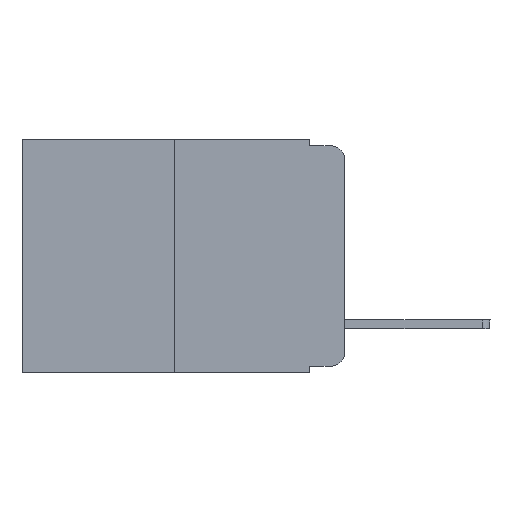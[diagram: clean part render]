
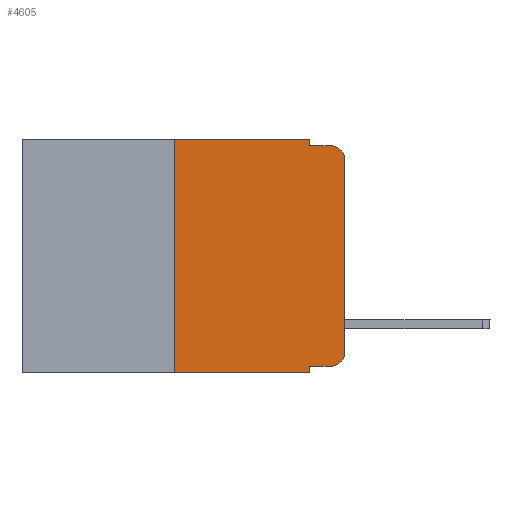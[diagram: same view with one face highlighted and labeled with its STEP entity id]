
A CAD part, left-side view. The second image highlights one B-rep face of the part: STEP entity #4605.
In plain terms, the highlighted planar face has unit normal (-1, 0, 0).
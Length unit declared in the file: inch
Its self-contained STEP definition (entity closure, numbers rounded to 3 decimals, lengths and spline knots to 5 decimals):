
#246 = CIRCLE ( 'NONE', #8995, 0.02 ) ;
#788 = LINE ( 'NONE', #16723, #5142 ) ;
#1160 = CARTESIAN_POINT ( 'NONE',  ( 0., 0.02, -0.01 ) ) ;
#1347 = AXIS2_PLACEMENT_3D ( 'NONE', #11598, #9607, #18611 ) ;
#1408 = FACE_OUTER_BOUND ( 'NONE', #2251, .T. ) ;
#1621 = CARTESIAN_POINT ( 'NONE',  ( 0., 0.25, 0. ) ) ;
#1906 = VECTOR ( 'NONE', #4057, 39.37008 ) ;
#2251 = EDGE_LOOP ( 'NONE', ( #18524, #17222, #21481, #17770, #9551, #10128, #10419, #15243, #20229, #13211 ) ) ;
#2508 = VECTOR ( 'NONE', #10291, 39.37008 ) ;
#2609 = DIRECTION ( 'NONE',  ( 0., 0., -1. ) ) ;
#3590 = VECTOR ( 'NONE', #8158, 39.37008 ) ;
#3754 = DIRECTION ( 'NONE',  ( -1., 0., 0. ) ) ;
#3791 = VERTEX_POINT ( 'NONE', #1160 ) ;
#4057 = DIRECTION ( 'NONE',  ( 0., -1., 0. ) ) ;
#4259 = VERTEX_POINT ( 'NONE', #8747 ) ;
#4409 = VECTOR ( 'NONE', #15600, 39.37008 ) ;
#4416 = LINE ( 'NONE', #5981, #1906 ) ;
#4605 = ADVANCED_FACE ( 'NONE', ( #1408 ), #8684, .F. ) ;
#4695 = LINE ( 'NONE', #9838, #3590 ) ;
#5142 = VECTOR ( 'NONE', #13490, 39.37008 ) ;
#5981 = CARTESIAN_POINT ( 'NONE',  ( 0., 0.051, -0.01 ) ) ;
#6121 = DIRECTION ( 'NONE',  ( 0., -1., 0. ) ) ;
#6798 = CARTESIAN_POINT ( 'NONE',  ( 0., 0.051, -0.01 ) ) ;
#7485 = VERTEX_POINT ( 'NONE', #21274 ) ;
#7593 = EDGE_CURVE ( 'NONE', #18343, #19414, #18879, .T. ) ;
#8158 = DIRECTION ( 'NONE',  ( 0., 0., -1. ) ) ;
#8684 = PLANE ( 'NONE',  #21352 ) ;
#8747 = CARTESIAN_POINT ( 'NONE',  ( 0., 0.02, -0.333 ) ) ;
#8995 = AXIS2_PLACEMENT_3D ( 'NONE', #20031, #3754, #11020 ) ;
#9551 = ORIENTED_EDGE ( 'NONE', *, *, #21444, .F. ) ;
#9607 = DIRECTION ( 'NONE',  ( -1., 0., 0. ) ) ;
#9838 = CARTESIAN_POINT ( 'NONE',  ( 0., 0.051, 0. ) ) ;
#10128 = ORIENTED_EDGE ( 'NONE', *, *, #14456, .F. ) ;
#10291 = DIRECTION ( 'NONE',  ( 0., -1., 0. ) ) ;
#10419 = ORIENTED_EDGE ( 'NONE', *, *, #19609, .T. ) ;
#10568 = VERTEX_POINT ( 'NONE', #11432 ) ;
#11020 = DIRECTION ( 'NONE',  ( 0., 0., -1. ) ) ;
#11432 = CARTESIAN_POINT ( 'NONE',  ( 0., 0., -0.313 ) ) ;
#11434 = EDGE_CURVE ( 'NONE', #19414, #3791, #4416, .T. ) ;
#11574 = CARTESIAN_POINT ( 'NONE',  ( 0., 0.051, -0.333 ) ) ;
#11598 = CARTESIAN_POINT ( 'NONE',  ( 0., 0.02, -0.03 ) ) ;
#11704 = VECTOR ( 'NONE', #2609, 39.37008 ) ;
#11774 = CARTESIAN_POINT ( 'NONE',  ( 0., 0.051, 0. ) ) ;
#12017 = CARTESIAN_POINT ( 'NONE',  ( 0., 0.25, 0. ) ) ;
#12063 = EDGE_CURVE ( 'NONE', #4259, #10568, #246, .T. ) ;
#12371 = CARTESIAN_POINT ( 'NONE',  ( 0., 0.473, -0.343 ) ) ;
#13091 = VERTEX_POINT ( 'NONE', #1621 ) ;
#13211 = ORIENTED_EDGE ( 'NONE', *, *, #12063, .T. ) ;
#13381 = EDGE_CURVE ( 'NONE', #22031, #3791, #15772, .T. ) ;
#13439 = EDGE_CURVE ( 'NONE', #10568, #22031, #788, .T. ) ;
#13490 = DIRECTION ( 'NONE',  ( 0., 0., 1. ) ) ;
#13846 = EDGE_CURVE ( 'NONE', #22821, #4259, #22510, .T. ) ;
#13919 = LINE ( 'NONE', #12017, #4409 ) ;
#14139 = DIRECTION ( 'NONE',  ( 0., 0., -1. ) ) ;
#14456 = EDGE_CURVE ( 'NONE', #7485, #13091, #13919, .T. ) ;
#15243 = ORIENTED_EDGE ( 'NONE', *, *, #18500, .F. ) ;
#15415 = LINE ( 'NONE', #12371, #2508 ) ;
#15416 = VECTOR ( 'NONE', #6121, 39.37008 ) ;
#15600 = DIRECTION ( 'NONE',  ( 0., 0., 1. ) ) ;
#15703 = VERTEX_POINT ( 'NONE', #16087 ) ;
#15772 = CIRCLE ( 'NONE', #1347, 0.02 ) ;
#15919 = CARTESIAN_POINT ( 'NONE',  ( 0., 0.473, 0. ) ) ;
#16087 = CARTESIAN_POINT ( 'NONE',  ( 0., 0.051, -0.343 ) ) ;
#16626 = CARTESIAN_POINT ( 'NONE',  ( 0., 0.473, 0. ) ) ;
#16723 = CARTESIAN_POINT ( 'NONE',  ( 0., 0., 0. ) ) ;
#17222 = ORIENTED_EDGE ( 'NONE', *, *, #13381, .T. ) ;
#17770 = ORIENTED_EDGE ( 'NONE', *, *, #7593, .F. ) ;
#18173 = LINE ( 'NONE', #16626, #21127 ) ;
#18343 = VERTEX_POINT ( 'NONE', #18358 ) ;
#18358 = CARTESIAN_POINT ( 'NONE',  ( 0., 0.051, 0. ) ) ;
#18500 = EDGE_CURVE ( 'NONE', #22821, #15703, #4695, .T. ) ;
#18524 = ORIENTED_EDGE ( 'NONE', *, *, #13439, .T. ) ;
#18611 = DIRECTION ( 'NONE',  ( 0., 0., -1. ) ) ;
#18879 = LINE ( 'NONE', #11774, #11704 ) ;
#19414 = VERTEX_POINT ( 'NONE', #6798 ) ;
#19609 = EDGE_CURVE ( 'NONE', #7485, #15703, #15415, .T. ) ;
#20031 = CARTESIAN_POINT ( 'NONE',  ( 0., 0.02, -0.313 ) ) ;
#20229 = ORIENTED_EDGE ( 'NONE', *, *, #13846, .T. ) ;
#20265 = CARTESIAN_POINT ( 'NONE',  ( 0., 0., -0.03 ) ) ;
#20289 = DIRECTION ( 'NONE',  ( 0., -1., 0. ) ) ;
#21127 = VECTOR ( 'NONE', #20289, 39.37008 ) ;
#21274 = CARTESIAN_POINT ( 'NONE',  ( 0., 0.25, -0.343 ) ) ;
#21352 = AXIS2_PLACEMENT_3D ( 'NONE', #15919, #23170, #14139 ) ;
#21444 = EDGE_CURVE ( 'NONE', #13091, #18343, #18173, .T. ) ;
#21481 = ORIENTED_EDGE ( 'NONE', *, *, #11434, .F. ) ;
#22031 = VERTEX_POINT ( 'NONE', #20265 ) ;
#22198 = CARTESIAN_POINT ( 'NONE',  ( 0., 0.051, -0.333 ) ) ;
#22510 = LINE ( 'NONE', #11574, #15416 ) ;
#22821 = VERTEX_POINT ( 'NONE', #22198 ) ;
#23170 = DIRECTION ( 'NONE',  ( 1., 0., 0. ) ) ;
